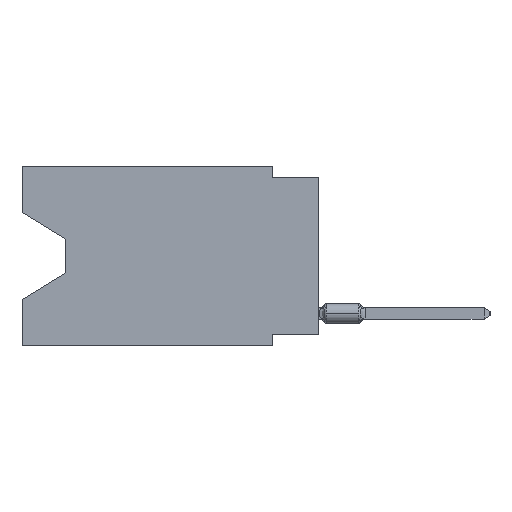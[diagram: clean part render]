
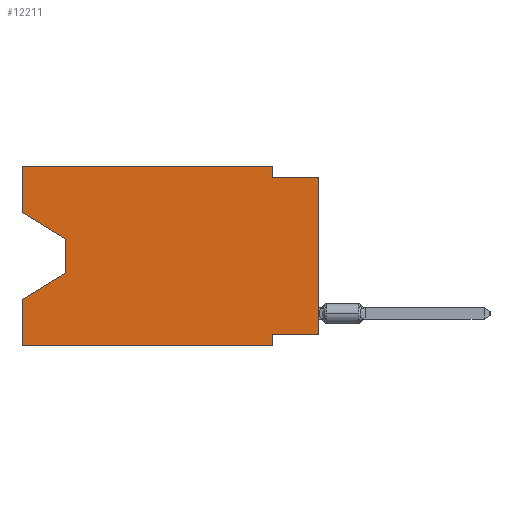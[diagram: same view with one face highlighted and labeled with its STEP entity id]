
A CAD part, left-side view. The second image highlights one B-rep face of the part: STEP entity #12211.
In plain terms, the highlighted planar face has unit normal (-1, 0, 0).
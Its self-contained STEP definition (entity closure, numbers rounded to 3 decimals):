
#1622 = VERTEX_POINT ( 'NONE', #17972 ) ;
#4362 = VERTEX_POINT ( 'NONE', #27136 ) ;
#5955 = LINE ( 'NONE', #25393, #75828 ) ;
#6053 = EDGE_LOOP ( 'NONE', ( #52419, #55742, #31979, #72306, #80903, #69959, #12510, #55834, #14341, #38795, #61382, #56836 ) ) ;
#7277 = LINE ( 'NONE', #41344, #69749 ) ;
#8313 = CARTESIAN_POINT ( 'NONE',  ( 0., 0., -0.635 ) ) ;
#8576 = VECTOR ( 'NONE', #25679, 1000. ) ;
#8923 = LINE ( 'NONE', #61626, #40209 ) ;
#9428 = CARTESIAN_POINT ( 'NONE',  ( 0., 0., -9.271 ) ) ;
#10086 = CARTESIAN_POINT ( 'NONE',  ( 0., 2.54, -9.906 ) ) ;
#10114 = LINE ( 'NONE', #75790, #60924 ) ;
#10164 = VERTEX_POINT ( 'NONE', #21274 ) ;
#10924 = DIRECTION ( 'NONE',  ( 0., -1., 0. ) ) ;
#11646 = LINE ( 'NONE', #82921, #78338 ) ;
#12150 = VECTOR ( 'NONE', #10924, 1000. ) ;
#12211 = ADVANCED_FACE ( 'NONE', ( #15199 ), #61856, .F. ) ;
#12510 = ORIENTED_EDGE ( 'NONE', *, *, #83302, .F. ) ;
#14199 = VERTEX_POINT ( 'NONE', #78572 ) ;
#14341 = ORIENTED_EDGE ( 'NONE', *, *, #61895, .F. ) ;
#15199 = FACE_OUTER_BOUND ( 'NONE', #6053, .T. ) ;
#17353 = DIRECTION ( 'NONE',  ( 0., -0.855, -0.519 ) ) ;
#17972 = CARTESIAN_POINT ( 'NONE',  ( 0., 16.383, -9.906 ) ) ;
#21274 = CARTESIAN_POINT ( 'NONE',  ( 0., 16.383, -7.36 ) ) ;
#24561 = CARTESIAN_POINT ( 'NONE',  ( 0., 13.97, -5.893 ) ) ;
#25041 = VERTEX_POINT ( 'NONE', #24561 ) ;
#25393 = CARTESIAN_POINT ( 'NONE',  ( 0., 13.97, -4.013 ) ) ;
#25679 = DIRECTION ( 'NONE',  ( 0., 0.855, -0.519 ) ) ;
#27136 = CARTESIAN_POINT ( 'NONE',  ( 0., 13.97, -4.013 ) ) ;
#27359 = EDGE_CURVE ( 'NONE', #4362, #25041, #5955, .T. ) ;
#27987 = DIRECTION ( 'NONE',  ( 0., 0., 1. ) ) ;
#28131 = EDGE_CURVE ( 'NONE', #1622, #10164, #51857, .T. ) ;
#28947 = VERTEX_POINT ( 'NONE', #32626 ) ;
#29536 = LINE ( 'NONE', #10086, #82829 ) ;
#30119 = VERTEX_POINT ( 'NONE', #71534 ) ;
#30660 = VERTEX_POINT ( 'NONE', #8313 ) ;
#30664 = DIRECTION ( 'NONE',  ( 0., -1., 0. ) ) ;
#31979 = ORIENTED_EDGE ( 'NONE', *, *, #77598, .T. ) ;
#32037 = LINE ( 'NONE', #45005, #32448 ) ;
#32448 = VECTOR ( 'NONE', #17353, 1000. ) ;
#32626 = CARTESIAN_POINT ( 'NONE',  ( 0., 16.383, -2.546 ) ) ;
#32793 = EDGE_CURVE ( 'NONE', #68515, #30660, #38430, .T. ) ;
#34770 = EDGE_CURVE ( 'NONE', #46676, #14199, #29536, .T. ) ;
#37108 = CARTESIAN_POINT ( 'NONE',  ( 0., 0., -9.271 ) ) ;
#37279 = LINE ( 'NONE', #49817, #12150 ) ;
#37300 = DIRECTION ( 'NONE',  ( 0., 0., -1. ) ) ;
#38430 = LINE ( 'NONE', #38867, #83344 ) ;
#38795 = ORIENTED_EDGE ( 'NONE', *, *, #66116, .F. ) ;
#38867 = CARTESIAN_POINT ( 'NONE',  ( 0., 0., 0. ) ) ;
#40209 = VECTOR ( 'NONE', #81485, 1000. ) ;
#41344 = CARTESIAN_POINT ( 'NONE',  ( 0., 16.383, 0. ) ) ;
#44889 = VECTOR ( 'NONE', #48333, 1000. ) ;
#45005 = CARTESIAN_POINT ( 'NONE',  ( 0., 16.383, -2.546 ) ) ;
#46676 = VERTEX_POINT ( 'NONE', #52445 ) ;
#46890 = CARTESIAN_POINT ( 'NONE',  ( 0., 16.383, 0. ) ) ;
#48333 = DIRECTION ( 'NONE',  ( 0., 1., 0. ) ) ;
#49579 = EDGE_CURVE ( 'NONE', #53281, #30119, #10114, .T. ) ;
#49817 = CARTESIAN_POINT ( 'NONE',  ( 0., 0., -0.635 ) ) ;
#51433 = CARTESIAN_POINT ( 'NONE',  ( 0., 16.383, 0. ) ) ;
#51857 = LINE ( 'NONE', #51433, #55699 ) ;
#52419 = ORIENTED_EDGE ( 'NONE', *, *, #70787, .T. ) ;
#52445 = CARTESIAN_POINT ( 'NONE',  ( 0., 2.54, -9.271 ) ) ;
#52702 = DIRECTION ( 'NONE',  ( 0., 0., 1. ) ) ;
#53281 = VERTEX_POINT ( 'NONE', #46890 ) ;
#55699 = VECTOR ( 'NONE', #52702, 1000. ) ;
#55742 = ORIENTED_EDGE ( 'NONE', *, *, #27359, .T. ) ;
#55834 = ORIENTED_EDGE ( 'NONE', *, *, #32793, .T. ) ;
#55838 = VERTEX_POINT ( 'NONE', #66110 ) ;
#56836 = ORIENTED_EDGE ( 'NONE', *, *, #57362, .F. ) ;
#57362 = EDGE_CURVE ( 'NONE', #28947, #53281, #7277, .T. ) ;
#59171 = DIRECTION ( 'NONE',  ( 0., 0., 1. ) ) ;
#59451 = EDGE_CURVE ( 'NONE', #1622, #14199, #11646, .T. ) ;
#60924 = VECTOR ( 'NONE', #76637, 1000. ) ;
#61022 = CARTESIAN_POINT ( 'NONE',  ( 0., 16.383, 0. ) ) ;
#61382 = ORIENTED_EDGE ( 'NONE', *, *, #49579, .F. ) ;
#61626 = CARTESIAN_POINT ( 'NONE',  ( 0., 2.54, 0. ) ) ;
#61856 = PLANE ( 'NONE',  #74047 ) ;
#61895 = EDGE_CURVE ( 'NONE', #55838, #30660, #37279, .T. ) ;
#66110 = CARTESIAN_POINT ( 'NONE',  ( 0., 2.54, -0.635 ) ) ;
#66116 = EDGE_CURVE ( 'NONE', #30119, #55838, #8923, .T. ) ;
#67479 = DIRECTION ( 'NONE',  ( 1., 0., 0. ) ) ;
#68515 = VERTEX_POINT ( 'NONE', #37108 ) ;
#69749 = VECTOR ( 'NONE', #27987, 1000. ) ;
#69959 = ORIENTED_EDGE ( 'NONE', *, *, #34770, .F. ) ;
#70787 = EDGE_CURVE ( 'NONE', #28947, #4362, #32037, .T. ) ;
#71534 = CARTESIAN_POINT ( 'NONE',  ( 0., 2.54, 0. ) ) ;
#72306 = ORIENTED_EDGE ( 'NONE', *, *, #28131, .F. ) ;
#73550 = DIRECTION ( 'NONE',  ( 0., 0., -1. ) ) ;
#74047 = AXIS2_PLACEMENT_3D ( 'NONE', #61022, #67479, #73550 ) ;
#74255 = LINE ( 'NONE', #9428, #44889 ) ;
#75790 = CARTESIAN_POINT ( 'NONE',  ( 0., 16.383, 0. ) ) ;
#75828 = VECTOR ( 'NONE', #78096, 1000. ) ;
#76637 = DIRECTION ( 'NONE',  ( 0., -1., 0. ) ) ;
#77535 = CARTESIAN_POINT ( 'NONE',  ( 0., 13.97, -5.893 ) ) ;
#77598 = EDGE_CURVE ( 'NONE', #25041, #10164, #79222, .T. ) ;
#78096 = DIRECTION ( 'NONE',  ( 0., 0., -1. ) ) ;
#78338 = VECTOR ( 'NONE', #30664, 1000. ) ;
#78572 = CARTESIAN_POINT ( 'NONE',  ( 0., 2.54, -9.906 ) ) ;
#79222 = LINE ( 'NONE', #77535, #8576 ) ;
#80903 = ORIENTED_EDGE ( 'NONE', *, *, #59451, .T. ) ;
#81485 = DIRECTION ( 'NONE',  ( 0., 0., -1. ) ) ;
#82829 = VECTOR ( 'NONE', #37300, 1000. ) ;
#82921 = CARTESIAN_POINT ( 'NONE',  ( 0., 16.383, -9.906 ) ) ;
#83302 = EDGE_CURVE ( 'NONE', #68515, #46676, #74255, .T. ) ;
#83344 = VECTOR ( 'NONE', #59171, 1000. ) ;
